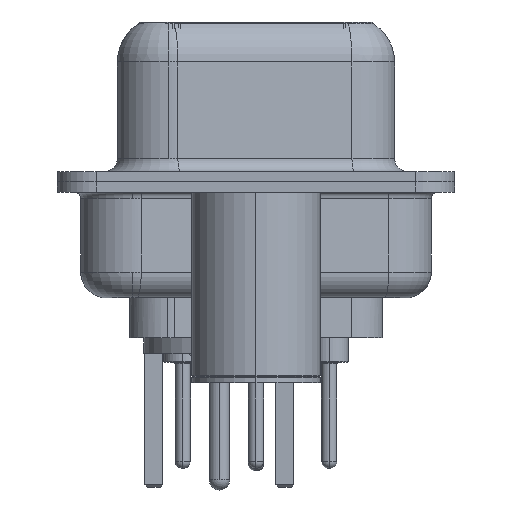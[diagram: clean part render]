
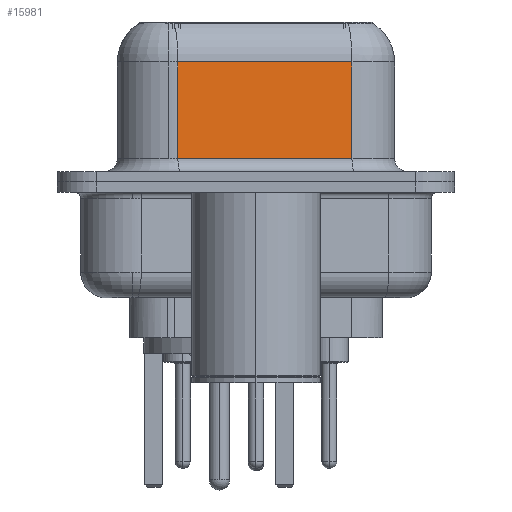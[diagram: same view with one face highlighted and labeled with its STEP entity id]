
A CAD part, left-side view. The second image highlights one B-rep face of the part: STEP entity #15981.
In plain terms, the highlighted planar face has unit normal (-0.985, -0.174, 0).
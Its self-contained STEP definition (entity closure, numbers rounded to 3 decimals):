
#480 = PLANE ( 'NONE',  #8081 ) ;
#1117 = DIRECTION ( 'NONE',  ( 0., 0., -1. ) ) ;
#2747 = ORIENTED_EDGE ( 'NONE', *, *, #27680, .T. ) ;
#2976 = VERTEX_POINT ( 'NONE', #33464 ) ;
#3195 = CARTESIAN_POINT ( 'NONE',  ( 5.621, -3.722, 6.4 ) ) ;
#3534 = CARTESIAN_POINT ( 'NONE',  ( 5.621, -3.722, 0.9 ) ) ;
#4328 = CARTESIAN_POINT ( 'NONE',  ( 5.621, -3.722, 6.4 ) ) ;
#5172 = VECTOR ( 'NONE', #9685, 1000. ) ;
#5743 = EDGE_CURVE ( 'NONE', #2976, #26653, #15563, .T. ) ;
#6658 = DIRECTION ( 'NONE',  ( 0.174, -0.985, 0. ) ) ;
#7080 = FACE_OUTER_BOUND ( 'NONE', #16107, .T. ) ;
#8081 = AXIS2_PLACEMENT_3D ( 'NONE', #3195, #14123, #24873 ) ;
#8476 = LINE ( 'NONE', #4328, #5172 ) ;
#9685 = DIRECTION ( 'NONE',  ( 0., 0., -1. ) ) ;
#12336 = CARTESIAN_POINT ( 'NONE',  ( 5.621, -3.722, 0.9 ) ) ;
#13041 = EDGE_CURVE ( 'NONE', #14264, #23831, #15536, .T. ) ;
#14123 = DIRECTION ( 'NONE',  ( 0.985, 0.174, 0. ) ) ;
#14264 = VERTEX_POINT ( 'NONE', #33170 ) ;
#14284 = CARTESIAN_POINT ( 'NONE',  ( 4.43, 3.028, 6.4 ) ) ;
#15536 = LINE ( 'NONE', #12336, #25144 ) ;
#15563 = LINE ( 'NONE', #19201, #28502 ) ;
#15981 = ADVANCED_FACE ( 'NONE', ( #7080 ), #480, .F. ) ;
#16107 = EDGE_LOOP ( 'NONE', ( #26332, #16336, #2747, #19239 ) ) ;
#16336 = ORIENTED_EDGE ( 'NONE', *, *, #5743, .T. ) ;
#16840 = DIRECTION ( 'NONE',  ( -0.174, 0.985, 0. ) ) ;
#19201 = CARTESIAN_POINT ( 'NONE',  ( 5.621, -3.722, 4.65 ) ) ;
#19239 = ORIENTED_EDGE ( 'NONE', *, *, #13041, .T. ) ;
#23831 = VERTEX_POINT ( 'NONE', #3534 ) ;
#24128 = EDGE_CURVE ( 'NONE', #2976, #23831, #8476, .T. ) ;
#24279 = LINE ( 'NONE', #14284, #29293 ) ;
#24873 = DIRECTION ( 'NONE',  ( -0.174, 0.985, 0. ) ) ;
#25144 = VECTOR ( 'NONE', #6658, 1000. ) ;
#26332 = ORIENTED_EDGE ( 'NONE', *, *, #24128, .F. ) ;
#26653 = VERTEX_POINT ( 'NONE', #28803 ) ;
#27680 = EDGE_CURVE ( 'NONE', #26653, #14264, #24279, .T. ) ;
#28502 = VECTOR ( 'NONE', #16840, 1000. ) ;
#28803 = CARTESIAN_POINT ( 'NONE',  ( 4.43, 3.028, 4.65 ) ) ;
#29293 = VECTOR ( 'NONE', #1117, 1000. ) ;
#33170 = CARTESIAN_POINT ( 'NONE',  ( 4.43, 3.028, 0.9 ) ) ;
#33464 = CARTESIAN_POINT ( 'NONE',  ( 5.621, -3.722, 4.65 ) ) ;
